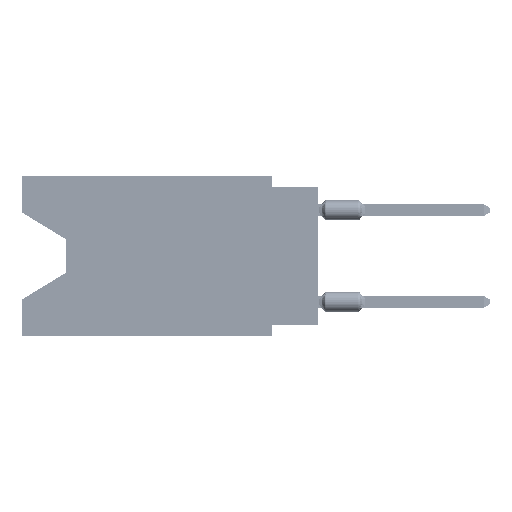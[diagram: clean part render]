
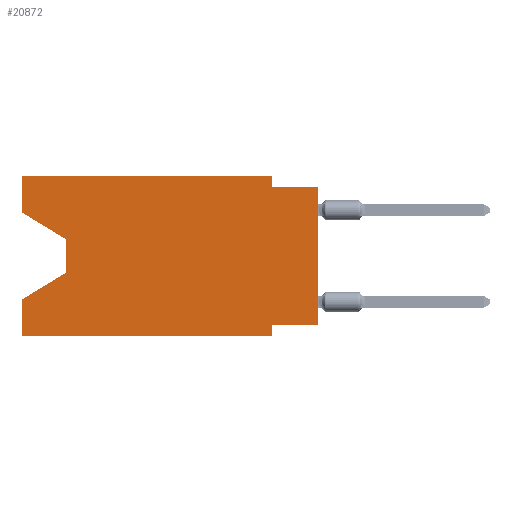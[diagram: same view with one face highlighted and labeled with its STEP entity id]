
A CAD part, left-side view. The second image highlights one B-rep face of the part: STEP entity #20872.
In plain terms, the highlighted planar face has unit normal (-1, 0, 0).
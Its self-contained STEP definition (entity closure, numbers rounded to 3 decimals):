
#1719 = CARTESIAN_POINT ( 'NONE',  ( 0., 16.383, -2.038 ) ) ;
#2585 = VERTEX_POINT ( 'NONE', #1719 ) ;
#3227 = VERTEX_POINT ( 'NONE', #40229 ) ;
#4496 = EDGE_CURVE ( 'NONE', #37981, #100894, #63514, .T. ) ;
#5180 = DIRECTION ( 'NONE',  ( 0., 1., 0. ) ) ;
#6907 = ORIENTED_EDGE ( 'NONE', *, *, #33541, .F. ) ;
#9572 = ORIENTED_EDGE ( 'NONE', *, *, #21035, .F. ) ;
#10824 = LINE ( 'NONE', #27731, #22788 ) ;
#11998 = CARTESIAN_POINT ( 'NONE',  ( 0., 16.383, 0. ) ) ;
#12413 = EDGE_CURVE ( 'NONE', #37981, #41427, #68886, .T. ) ;
#14023 = ORIENTED_EDGE ( 'NONE', *, *, #12413, .T. ) ;
#14846 = DIRECTION ( 'NONE',  ( 0., 0., -1. ) ) ;
#16541 = EDGE_CURVE ( 'NONE', #38149, #106957, #54847, .T. ) ;
#17937 = LINE ( 'NONE', #41920, #84900 ) ;
#19472 = VECTOR ( 'NONE', #14846, 1000. ) ;
#20076 = CARTESIAN_POINT ( 'NONE',  ( 0., 16.383, -8.89 ) ) ;
#20872 = ADVANCED_FACE ( 'NONE', ( #78543 ), #70365, .F. ) ;
#21035 = EDGE_CURVE ( 'NONE', #70214, #41427, #17937, .T. ) ;
#21461 = CARTESIAN_POINT ( 'NONE',  ( 0., 16.383, -8.89 ) ) ;
#22411 = CARTESIAN_POINT ( 'NONE',  ( 0., 16.383, 0. ) ) ;
#22788 = VECTOR ( 'NONE', #69165, 1000. ) ;
#23090 = CARTESIAN_POINT ( 'NONE',  ( 0., 13.97, -3.505 ) ) ;
#24034 = DIRECTION ( 'NONE',  ( 0., -1., 0. ) ) ;
#24532 = CARTESIAN_POINT ( 'NONE',  ( 0., 13.97, -5.385 ) ) ;
#25039 = VECTOR ( 'NONE', #79946, 1000. ) ;
#25162 = VECTOR ( 'NONE', #5180, 1000. ) ;
#27466 = DIRECTION ( 'NONE',  ( 0., 0., 1. ) ) ;
#27731 = CARTESIAN_POINT ( 'NONE',  ( 0., 16.383, 0. ) ) ;
#29457 = DIRECTION ( 'NONE',  ( 0., 0., -1. ) ) ;
#29869 = DIRECTION ( 'NONE',  ( 0., 0., -1. ) ) ;
#30266 = CARTESIAN_POINT ( 'NONE',  ( 0., 0., -8.255 ) ) ;
#33087 = VERTEX_POINT ( 'NONE', #51295 ) ;
#33541 = EDGE_CURVE ( 'NONE', #2585, #91618, #10824, .T. ) ;
#33582 = EDGE_CURVE ( 'NONE', #76504, #38149, #53856, .T. ) ;
#34698 = ORIENTED_EDGE ( 'NONE', *, *, #94974, .T. ) ;
#35497 = CARTESIAN_POINT ( 'NONE',  ( 0., 0., -0.635 ) ) ;
#37981 = VERTEX_POINT ( 'NONE', #63784 ) ;
#38149 = VERTEX_POINT ( 'NONE', #24532 ) ;
#40229 = CARTESIAN_POINT ( 'NONE',  ( 0., 2.54, -8.89 ) ) ;
#41427 = VERTEX_POINT ( 'NONE', #35497 ) ;
#41920 = CARTESIAN_POINT ( 'NONE',  ( 0., 0., -0.635 ) ) ;
#43799 = LINE ( 'NONE', #77078, #19472 ) ;
#44964 = ORIENTED_EDGE ( 'NONE', *, *, #4496, .F. ) ;
#46669 = CARTESIAN_POINT ( 'NONE',  ( 0., 13.97, -5.385 ) ) ;
#50625 = DIRECTION ( 'NONE',  ( 0., -1., 0. ) ) ;
#51295 = CARTESIAN_POINT ( 'NONE',  ( 0., 2.54, 0. ) ) ;
#53856 = LINE ( 'NONE', #87146, #78515 ) ;
#54847 = LINE ( 'NONE', #46669, #25039 ) ;
#55133 = VECTOR ( 'NONE', #86187, 1000. ) ;
#56770 = VECTOR ( 'NONE', #102661, 1000. ) ;
#61736 = LINE ( 'NONE', #77042, #56770 ) ;
#62762 = ORIENTED_EDGE ( 'NONE', *, *, #83058, .F. ) ;
#63043 = DIRECTION ( 'NONE',  ( 0., 0., -1. ) ) ;
#63314 = LINE ( 'NONE', #22411, #102647 ) ;
#63514 = LINE ( 'NONE', #30266, #25162 ) ;
#63784 = CARTESIAN_POINT ( 'NONE',  ( 0., 0., -8.255 ) ) ;
#66922 = VECTOR ( 'NONE', #63043, 1000. ) ;
#68886 = LINE ( 'NONE', #102165, #102754 ) ;
#69165 = DIRECTION ( 'NONE',  ( 0., 0., 1. ) ) ;
#70214 = VERTEX_POINT ( 'NONE', #103362 ) ;
#70365 = PLANE ( 'NONE',  #104027 ) ;
#71086 = DIRECTION ( 'NONE',  ( 0., -1., 0. ) ) ;
#72986 = ORIENTED_EDGE ( 'NONE', *, *, #85371, .F. ) ;
#74608 = CARTESIAN_POINT ( 'NONE',  ( 0., 2.54, -8.255 ) ) ;
#75924 = ORIENTED_EDGE ( 'NONE', *, *, #101152, .F. ) ;
#76504 = VERTEX_POINT ( 'NONE', #23090 ) ;
#76921 = LINE ( 'NONE', #11998, #55133 ) ;
#77042 = CARTESIAN_POINT ( 'NONE',  ( 0., 16.383, -2.038 ) ) ;
#77078 = CARTESIAN_POINT ( 'NONE',  ( 0., 2.54, 0. ) ) ;
#78515 = VECTOR ( 'NONE', #29869, 1000. ) ;
#78543 = FACE_OUTER_BOUND ( 'NONE', #88555, .T. ) ;
#78729 = LINE ( 'NONE', #21461, #80008 ) ;
#78881 = CARTESIAN_POINT ( 'NONE',  ( 0., 2.54, -8.89 ) ) ;
#79946 = DIRECTION ( 'NONE',  ( 0., 0.855, -0.519 ) ) ;
#80008 = VECTOR ( 'NONE', #71086, 1000. ) ;
#81305 = ORIENTED_EDGE ( 'NONE', *, *, #97048, .F. ) ;
#83058 = EDGE_CURVE ( 'NONE', #105095, #106957, #76921, .T. ) ;
#84900 = VECTOR ( 'NONE', #50625, 1000. ) ;
#85371 = EDGE_CURVE ( 'NONE', #91618, #33087, #63314, .T. ) ;
#86187 = DIRECTION ( 'NONE',  ( 0., 0., 1. ) ) ;
#87146 = CARTESIAN_POINT ( 'NONE',  ( 0., 13.97, -3.505 ) ) ;
#87625 = ORIENTED_EDGE ( 'NONE', *, *, #33582, .T. ) ;
#88555 = EDGE_LOOP ( 'NONE', ( #105363, #87625, #98935, #62762, #34698, #75924, #44964, #14023, #9572, #81305, #72986, #6907 ) ) ;
#89231 = LINE ( 'NONE', #78881, #66922 ) ;
#91618 = VERTEX_POINT ( 'NONE', #100421 ) ;
#91957 = CARTESIAN_POINT ( 'NONE',  ( 0., 16.383, -6.852 ) ) ;
#92060 = EDGE_CURVE ( 'NONE', #2585, #76504, #61736, .T. ) ;
#94974 = EDGE_CURVE ( 'NONE', #105095, #3227, #78729, .T. ) ;
#97048 = EDGE_CURVE ( 'NONE', #33087, #70214, #43799, .T. ) ;
#98935 = ORIENTED_EDGE ( 'NONE', *, *, #16541, .T. ) ;
#100421 = CARTESIAN_POINT ( 'NONE',  ( 0., 16.383, 0. ) ) ;
#100894 = VERTEX_POINT ( 'NONE', #74608 ) ;
#101152 = EDGE_CURVE ( 'NONE', #100894, #3227, #89231, .T. ) ;
#102165 = CARTESIAN_POINT ( 'NONE',  ( 0., 0., 0. ) ) ;
#102647 = VECTOR ( 'NONE', #24034, 1000. ) ;
#102661 = DIRECTION ( 'NONE',  ( 0., -0.855, -0.519 ) ) ;
#102754 = VECTOR ( 'NONE', #27466, 1000. ) ;
#103362 = CARTESIAN_POINT ( 'NONE',  ( 0., 2.54, -0.635 ) ) ;
#103637 = CARTESIAN_POINT ( 'NONE',  ( 0., 16.383, 0. ) ) ;
#104027 = AXIS2_PLACEMENT_3D ( 'NONE', #103637, #104162, #29457 ) ;
#104162 = DIRECTION ( 'NONE',  ( 1., 0., 0. ) ) ;
#105095 = VERTEX_POINT ( 'NONE', #20076 ) ;
#105363 = ORIENTED_EDGE ( 'NONE', *, *, #92060, .T. ) ;
#106957 = VERTEX_POINT ( 'NONE', #91957 ) ;
